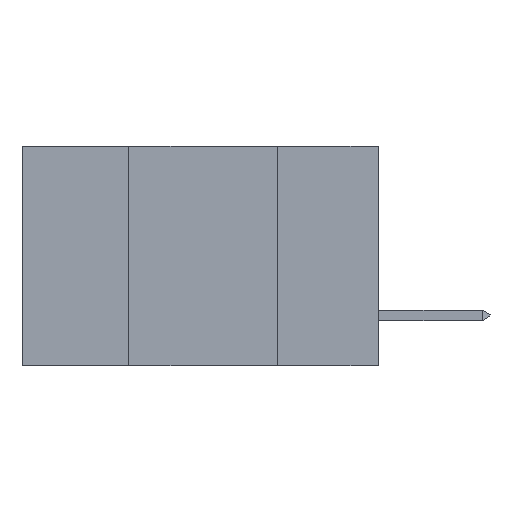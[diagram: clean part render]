
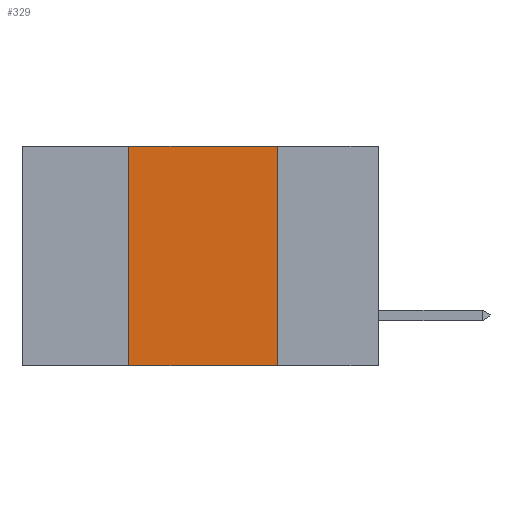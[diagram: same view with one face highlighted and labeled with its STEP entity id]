
A CAD part, left-side view. The second image highlights one B-rep face of the part: STEP entity #329.
In plain terms, the highlighted planar face has unit normal (-1, 0, 0).
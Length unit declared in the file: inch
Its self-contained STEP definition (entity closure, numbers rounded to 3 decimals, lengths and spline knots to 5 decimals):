
#329 = ADVANCED_FACE ( 'NONE', ( #20730 ), #26370, .F. ) ;
#2945 = VECTOR ( 'NONE', #22911, 39.37008 ) ;
#4822 = CARTESIAN_POINT ( 'NONE',  ( 0., 0.6, 0. ) ) ;
#5663 = ORIENTED_EDGE ( 'NONE', *, *, #6634, .F. ) ;
#6634 = EDGE_CURVE ( 'NONE', #26691, #14600, #20877, .T. ) ;
#7095 = DIRECTION ( 'NONE',  ( 1., 0., 0. ) ) ;
#7807 = CARTESIAN_POINT ( 'NONE',  ( 0., 0.6, -0.37 ) ) ;
#7868 = LINE ( 'NONE', #27053, #2945 ) ;
#8527 = CARTESIAN_POINT ( 'NONE',  ( 0., 0.42, 0. ) ) ;
#9538 = CARTESIAN_POINT ( 'NONE',  ( 0., 0.42, 0. ) ) ;
#10433 = ORIENTED_EDGE ( 'NONE', *, *, #21067, .F. ) ;
#10440 = LINE ( 'NONE', #9538, #18642 ) ;
#11168 = EDGE_CURVE ( 'NONE', #14600, #16653, #7868, .T. ) ;
#12025 = VECTOR ( 'NONE', #14153, 39.37008 ) ;
#13748 = DIRECTION ( 'NONE',  ( 0., 0., 1. ) ) ;
#14153 = DIRECTION ( 'NONE',  ( 0., -1., 0. ) ) ;
#14600 = VERTEX_POINT ( 'NONE', #22781 ) ;
#14903 = VERTEX_POINT ( 'NONE', #27017 ) ;
#15801 = AXIS2_PLACEMENT_3D ( 'NONE', #4822, #7095, #21555 ) ;
#16653 = VERTEX_POINT ( 'NONE', #23382 ) ;
#17003 = EDGE_CURVE ( 'NONE', #14903, #16653, #23771, .T. ) ;
#17342 = CARTESIAN_POINT ( 'NONE',  ( 0., 0.6, 0. ) ) ;
#18642 = VECTOR ( 'NONE', #13748, 39.37008 ) ;
#19413 = DIRECTION ( 'NONE',  ( 0., -1., 0. ) ) ;
#20224 = VECTOR ( 'NONE', #19413, 39.37008 ) ;
#20711 = ORIENTED_EDGE ( 'NONE', *, *, #17003, .T. ) ;
#20730 = FACE_OUTER_BOUND ( 'NONE', #23090, .T. ) ;
#20877 = LINE ( 'NONE', #17342, #20224 ) ;
#21067 = EDGE_CURVE ( 'NONE', #14903, #26691, #10440, .T. ) ;
#21555 = DIRECTION ( 'NONE',  ( 0., 0., -1. ) ) ;
#22562 = ORIENTED_EDGE ( 'NONE', *, *, #11168, .F. ) ;
#22781 = CARTESIAN_POINT ( 'NONE',  ( 0., 0.17, 0. ) ) ;
#22911 = DIRECTION ( 'NONE',  ( 0., 0., -1. ) ) ;
#23090 = EDGE_LOOP ( 'NONE', ( #22562, #5663, #10433, #20711 ) ) ;
#23382 = CARTESIAN_POINT ( 'NONE',  ( 0., 0.17, -0.37 ) ) ;
#23771 = LINE ( 'NONE', #7807, #12025 ) ;
#26370 = PLANE ( 'NONE',  #15801 ) ;
#26691 = VERTEX_POINT ( 'NONE', #8527 ) ;
#27017 = CARTESIAN_POINT ( 'NONE',  ( 0., 0.42, -0.37 ) ) ;
#27053 = CARTESIAN_POINT ( 'NONE',  ( 0., 0.17, 0. ) ) ;
